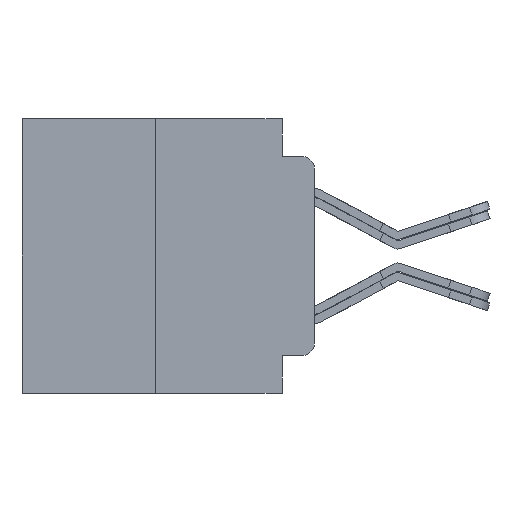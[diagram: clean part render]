
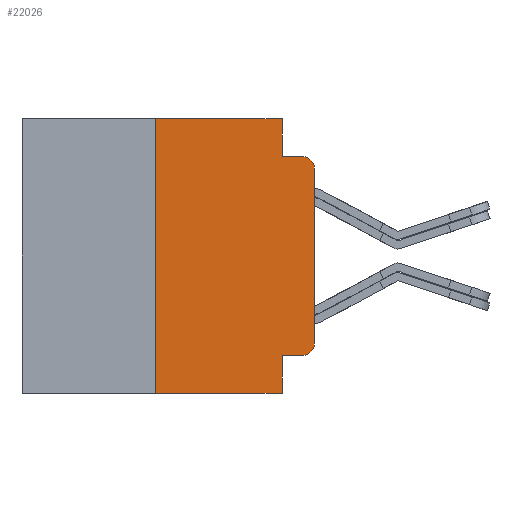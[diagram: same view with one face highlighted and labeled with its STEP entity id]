
A CAD part, left-side view. The second image highlights one B-rep face of the part: STEP entity #22026.
In plain terms, the highlighted planar face has unit normal (-1, 0, 0).
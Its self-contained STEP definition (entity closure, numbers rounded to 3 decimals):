
#195 = ORIENTED_EDGE ( 'NONE', *, *, #15109, .T. ) ;
#361 = ORIENTED_EDGE ( 'NONE', *, *, #4731, .T. ) ;
#638 = DIRECTION ( 'NONE',  ( 1., 0., 0. ) ) ;
#1045 = CARTESIAN_POINT ( 'NONE',  ( -75.603, 1.295, 3.975 ) ) ;
#1303 = DIRECTION ( 'NONE',  ( -1., 0., 0. ) ) ;
#1397 = DIRECTION ( 'NONE',  ( 0., 0., -1. ) ) ;
#1886 = CARTESIAN_POINT ( 'NONE',  ( -75.603, 6.35, -5.486 ) ) ;
#2074 = DIRECTION ( 'NONE',  ( 0., 0., -1. ) ) ;
#2412 = LINE ( 'NONE', #16359, #12870 ) ;
#2700 = PLANE ( 'NONE',  #22862 ) ;
#3008 = EDGE_CURVE ( 'NONE', #19431, #27556, #3735, .T. ) ;
#3013 = CARTESIAN_POINT ( 'NONE',  ( -75.603, 1.295, 5.486 ) ) ;
#3214 = VERTEX_POINT ( 'NONE', #20579 ) ;
#3735 = LINE ( 'NONE', #1886, #8344 ) ;
#3945 = ORIENTED_EDGE ( 'NONE', *, *, #23534, .F. ) ;
#4128 = FACE_OUTER_BOUND ( 'NONE', #22867, .T. ) ;
#4176 = VERTEX_POINT ( 'NONE', #14454 ) ;
#4401 = ORIENTED_EDGE ( 'NONE', *, *, #10240, .T. ) ;
#4731 = EDGE_CURVE ( 'NONE', #5729, #21310, #17826, .T. ) ;
#4831 = VECTOR ( 'NONE', #11011, 1000. ) ;
#5729 = VERTEX_POINT ( 'NONE', #20612 ) ;
#6071 = CARTESIAN_POINT ( 'NONE',  ( -75.603, 1.295, -5.486 ) ) ;
#6092 = VERTEX_POINT ( 'NONE', #14988 ) ;
#6443 = AXIS2_PLACEMENT_3D ( 'NONE', #21573, #1303, #1397 ) ;
#6561 = EDGE_CURVE ( 'NONE', #19431, #11707, #15273, .T. ) ;
#6798 = CARTESIAN_POINT ( 'NONE',  ( -75.603, 11.684, 5.486 ) ) ;
#7199 = DIRECTION ( 'NONE',  ( 0., -1., 0. ) ) ;
#7266 = CARTESIAN_POINT ( 'NONE',  ( -75.603, 0.508, 3.467 ) ) ;
#7445 = CARTESIAN_POINT ( 'NONE',  ( -75.603, 11.684, 5.486 ) ) ;
#7734 = VECTOR ( 'NONE', #2074, 1000. ) ;
#7797 = LINE ( 'NONE', #6798, #23921 ) ;
#7927 = LINE ( 'NONE', #1045, #12111 ) ;
#8344 = VECTOR ( 'NONE', #24221, 1000. ) ;
#8631 = EDGE_CURVE ( 'NONE', #24132, #6092, #12403, .T. ) ;
#9512 = DIRECTION ( 'NONE',  ( -1., 0., 0. ) ) ;
#9803 = DIRECTION ( 'NONE',  ( 0., -1., 0. ) ) ;
#10092 = CARTESIAN_POINT ( 'NONE',  ( -75.603, 6.35, -5.486 ) ) ;
#10111 = CARTESIAN_POINT ( 'NONE',  ( -75.603, 0., 5.486 ) ) ;
#10240 = EDGE_CURVE ( 'NONE', #18901, #4176, #2412, .T. ) ;
#11011 = DIRECTION ( 'NONE',  ( 0., 0., 1. ) ) ;
#11228 = EDGE_CURVE ( 'NONE', #4176, #3214, #19796, .T. ) ;
#11707 = VERTEX_POINT ( 'NONE', #6071 ) ;
#12111 = VECTOR ( 'NONE', #20927, 1000. ) ;
#12403 = LINE ( 'NONE', #13069, #27873 ) ;
#12741 = ORIENTED_EDGE ( 'NONE', *, *, #6561, .T. ) ;
#12795 = CARTESIAN_POINT ( 'NONE',  ( -75.603, 0.508, 3.975 ) ) ;
#12870 = VECTOR ( 'NONE', #9803, 1000. ) ;
#13069 = CARTESIAN_POINT ( 'NONE',  ( -75.603, 1.295, 0. ) ) ;
#13451 = ORIENTED_EDGE ( 'NONE', *, *, #27342, .F. ) ;
#14454 = CARTESIAN_POINT ( 'NONE',  ( -75.603, 0.508, -3.975 ) ) ;
#14817 = EDGE_CURVE ( 'NONE', #18901, #11707, #20707, .T. ) ;
#14988 = CARTESIAN_POINT ( 'NONE',  ( -75.603, 1.295, 3.975 ) ) ;
#14995 = DIRECTION ( 'NONE',  ( 0., -1., 0. ) ) ;
#15109 = EDGE_CURVE ( 'NONE', #3214, #5729, #18200, .T. ) ;
#15273 = LINE ( 'NONE', #19774, #22684 ) ;
#15481 = CARTESIAN_POINT ( 'NONE',  ( -75.603, 1.295, -3.975 ) ) ;
#15547 = CARTESIAN_POINT ( 'NONE',  ( -75.603, 1.295, 0. ) ) ;
#16359 = CARTESIAN_POINT ( 'NONE',  ( -75.603, 1.295, -3.975 ) ) ;
#16901 = DIRECTION ( 'NONE',  ( 0., 0., -1. ) ) ;
#17826 = CIRCLE ( 'NONE', #26131, 0.508 ) ;
#18200 = LINE ( 'NONE', #10111, #4831 ) ;
#18575 = ORIENTED_EDGE ( 'NONE', *, *, #3008, .F. ) ;
#18901 = VERTEX_POINT ( 'NONE', #15481 ) ;
#19431 = VERTEX_POINT ( 'NONE', #10092 ) ;
#19774 = CARTESIAN_POINT ( 'NONE',  ( -75.603, 11.684, -5.486 ) ) ;
#19796 = CIRCLE ( 'NONE', #6443, 0.508 ) ;
#20579 = CARTESIAN_POINT ( 'NONE',  ( -75.603, 0., -3.467 ) ) ;
#20612 = CARTESIAN_POINT ( 'NONE',  ( -75.603, 0., 3.467 ) ) ;
#20707 = LINE ( 'NONE', #15547, #7734 ) ;
#20927 = DIRECTION ( 'NONE',  ( 0., -1., 0. ) ) ;
#21310 = VERTEX_POINT ( 'NONE', #12795 ) ;
#21573 = CARTESIAN_POINT ( 'NONE',  ( -75.603, 0.508, -3.467 ) ) ;
#22023 = DIRECTION ( 'NONE',  ( 0., 0., -1. ) ) ;
#22026 = ADVANCED_FACE ( 'NONE', ( #4128 ), #2700, .F. ) ;
#22684 = VECTOR ( 'NONE', #14995, 1000. ) ;
#22862 = AXIS2_PLACEMENT_3D ( 'NONE', #7445, #638, #23152 ) ;
#22867 = EDGE_LOOP ( 'NONE', ( #4401, #26210, #195, #361, #3945, #23415, #13451, #18575, #12741, #27395 ) ) ;
#23152 = DIRECTION ( 'NONE',  ( 0., 0., -1. ) ) ;
#23415 = ORIENTED_EDGE ( 'NONE', *, *, #8631, .F. ) ;
#23534 = EDGE_CURVE ( 'NONE', #6092, #21310, #7927, .T. ) ;
#23921 = VECTOR ( 'NONE', #7199, 1000. ) ;
#24132 = VERTEX_POINT ( 'NONE', #3013 ) ;
#24221 = DIRECTION ( 'NONE',  ( 0., 0., 1. ) ) ;
#26131 = AXIS2_PLACEMENT_3D ( 'NONE', #7266, #9512, #16901 ) ;
#26210 = ORIENTED_EDGE ( 'NONE', *, *, #11228, .T. ) ;
#27342 = EDGE_CURVE ( 'NONE', #27556, #24132, #7797, .T. ) ;
#27395 = ORIENTED_EDGE ( 'NONE', *, *, #14817, .F. ) ;
#27556 = VERTEX_POINT ( 'NONE', #27805 ) ;
#27805 = CARTESIAN_POINT ( 'NONE',  ( -75.603, 6.35, 5.486 ) ) ;
#27873 = VECTOR ( 'NONE', #22023, 1000. ) ;
